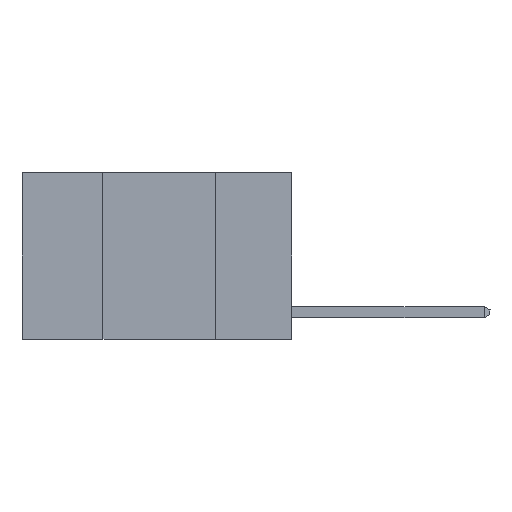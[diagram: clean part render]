
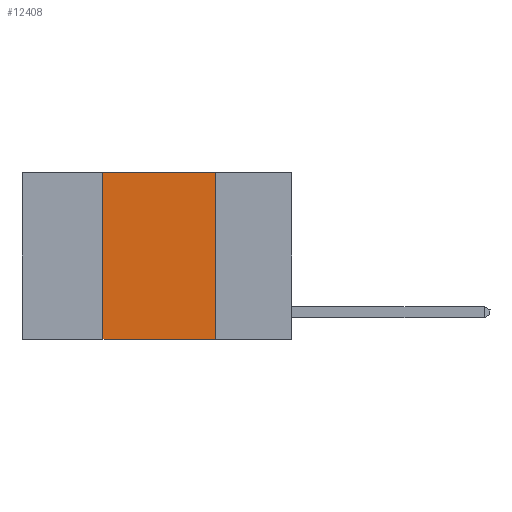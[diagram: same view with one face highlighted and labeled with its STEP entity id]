
A CAD part, left-side view. The second image highlights one B-rep face of the part: STEP entity #12408.
In plain terms, the highlighted planar face has unit normal (-1, 0, 0).
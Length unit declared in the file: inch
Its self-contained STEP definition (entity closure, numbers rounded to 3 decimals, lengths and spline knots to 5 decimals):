
#1671 = VECTOR ( 'NONE', #3937, 39.37008 ) ;
#1894 = CARTESIAN_POINT ( 'NONE',  ( 0., 0.42, 0. ) ) ;
#1942 = CARTESIAN_POINT ( 'NONE',  ( 0., 0.6, 0. ) ) ;
#2184 = DIRECTION ( 'NONE',  ( 1., 0., 0. ) ) ;
#2194 = LINE ( 'NONE', #1894, #14561 ) ;
#2760 = ORIENTED_EDGE ( 'NONE', *, *, #12956, .T. ) ;
#3465 = EDGE_CURVE ( 'NONE', #12019, #8593, #10928, .T. ) ;
#3937 = DIRECTION ( 'NONE',  ( 0., 0., -1. ) ) ;
#4023 = VECTOR ( 'NONE', #5437, 39.37008 ) ;
#5437 = DIRECTION ( 'NONE',  ( 0., -1., 0. ) ) ;
#5617 = DIRECTION ( 'NONE',  ( 0., -1., 0. ) ) ;
#6329 = ORIENTED_EDGE ( 'NONE', *, *, #14301, .F. ) ;
#6339 = EDGE_CURVE ( 'NONE', #8631, #12019, #2194, .T. ) ;
#6432 = FACE_OUTER_BOUND ( 'NONE', #11135, .T. ) ;
#6638 = DIRECTION ( 'NONE',  ( 0., 0., 1. ) ) ;
#6926 = PLANE ( 'NONE',  #7277 ) ;
#7277 = AXIS2_PLACEMENT_3D ( 'NONE', #10699, #2184, #14078 ) ;
#8593 = VERTEX_POINT ( 'NONE', #15164 ) ;
#8631 = VERTEX_POINT ( 'NONE', #13555 ) ;
#9880 = CARTESIAN_POINT ( 'NONE',  ( 0., 0.17, 0. ) ) ;
#10332 = CARTESIAN_POINT ( 'NONE',  ( 0., 0.6, -0.37 ) ) ;
#10417 = ORIENTED_EDGE ( 'NONE', *, *, #6339, .F. ) ;
#10660 = CARTESIAN_POINT ( 'NONE',  ( 0., 0.42, 0. ) ) ;
#10699 = CARTESIAN_POINT ( 'NONE',  ( 0., 0.6, 0. ) ) ;
#10928 = LINE ( 'NONE', #1942, #4023 ) ;
#11135 = EDGE_LOOP ( 'NONE', ( #6329, #11605, #10417, #2760 ) ) ;
#11605 = ORIENTED_EDGE ( 'NONE', *, *, #3465, .F. ) ;
#12019 = VERTEX_POINT ( 'NONE', #10660 ) ;
#12408 = ADVANCED_FACE ( 'NONE', ( #6432 ), #6926, .F. ) ;
#12956 = EDGE_CURVE ( 'NONE', #8631, #14949, #15190, .T. ) ;
#13249 = CARTESIAN_POINT ( 'NONE',  ( 0., 0.17, -0.37 ) ) ;
#13504 = VECTOR ( 'NONE', #5617, 39.37008 ) ;
#13555 = CARTESIAN_POINT ( 'NONE',  ( 0., 0.42, -0.37 ) ) ;
#14078 = DIRECTION ( 'NONE',  ( 0., 0., -1. ) ) ;
#14301 = EDGE_CURVE ( 'NONE', #8593, #14949, #14568, .T. ) ;
#14561 = VECTOR ( 'NONE', #6638, 39.37008 ) ;
#14568 = LINE ( 'NONE', #9880, #1671 ) ;
#14949 = VERTEX_POINT ( 'NONE', #13249 ) ;
#15164 = CARTESIAN_POINT ( 'NONE',  ( 0., 0.17, 0. ) ) ;
#15190 = LINE ( 'NONE', #10332, #13504 ) ;
